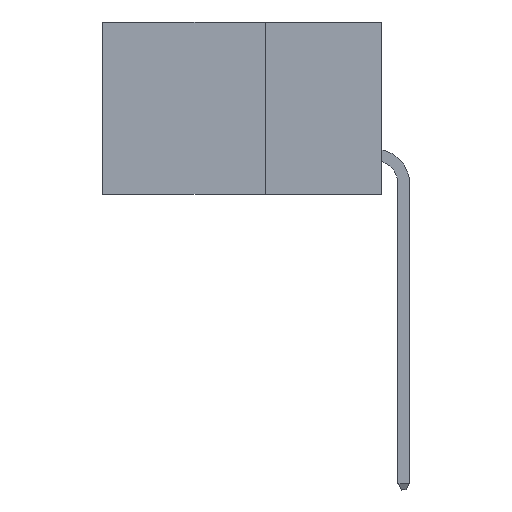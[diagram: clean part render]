
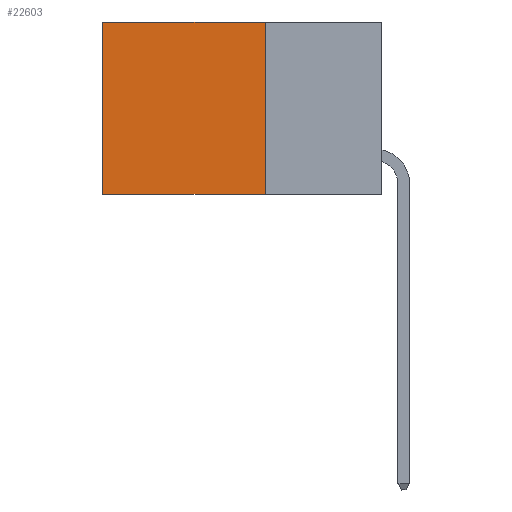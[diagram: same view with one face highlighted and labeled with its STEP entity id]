
A CAD part, left-side view. The second image highlights one B-rep face of the part: STEP entity #22603.
In plain terms, the highlighted planar face has unit normal (-1, 0, 0).
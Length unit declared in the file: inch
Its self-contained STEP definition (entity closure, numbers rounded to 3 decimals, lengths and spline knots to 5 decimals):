
#535 = VERTEX_POINT ( 'NONE', #19764 ) ;
#2864 = AXIS2_PLACEMENT_3D ( 'NONE', #6429, #10647, #20541 ) ;
#3341 = VECTOR ( 'NONE', #6551, 39.37008 ) ;
#3945 = VECTOR ( 'NONE', #6868, 39.37008 ) ;
#5042 = ORIENTED_EDGE ( 'NONE', *, *, #19455, .T. ) ;
#6429 = CARTESIAN_POINT ( 'NONE',  ( 0.2875, 0.25, 0. ) ) ;
#6497 = EDGE_CURVE ( 'NONE', #6923, #14140, #11892, .T. ) ;
#6551 = DIRECTION ( 'NONE',  ( 0., 0., -1. ) ) ;
#6698 = LINE ( 'NONE', #15968, #17803 ) ;
#6842 = CARTESIAN_POINT ( 'NONE',  ( 0.2875, 0.6, -0.37 ) ) ;
#6868 = DIRECTION ( 'NONE',  ( 0., 1., 0. ) ) ;
#6923 = VERTEX_POINT ( 'NONE', #15298 ) ;
#6982 = CARTESIAN_POINT ( 'NONE',  ( 0.2875, 0.25, 0. ) ) ;
#8754 = CARTESIAN_POINT ( 'NONE',  ( 0.2875, 0.25, 0. ) ) ;
#8800 = PLANE ( 'NONE',  #2864 ) ;
#9365 = CARTESIAN_POINT ( 'NONE',  ( 0.2875, 0.25, -0.37 ) ) ;
#10647 = DIRECTION ( 'NONE',  ( 1., 0., 0. ) ) ;
#11892 = LINE ( 'NONE', #9365, #3945 ) ;
#12185 = VERTEX_POINT ( 'NONE', #6982 ) ;
#14140 = VERTEX_POINT ( 'NONE', #6842 ) ;
#15125 = ORIENTED_EDGE ( 'NONE', *, *, #24851, .F. ) ;
#15298 = CARTESIAN_POINT ( 'NONE',  ( 0.2875, 0.25, -0.37 ) ) ;
#15968 = CARTESIAN_POINT ( 'NONE',  ( 0.2875, 0.25, 0. ) ) ;
#17476 = DIRECTION ( 'NONE',  ( 0., 0., -1. ) ) ;
#17803 = VECTOR ( 'NONE', #23981, 39.37008 ) ;
#19455 = EDGE_CURVE ( 'NONE', #535, #14140, #25986, .T. ) ;
#19461 = LINE ( 'NONE', #8754, #3341 ) ;
#19558 = FACE_OUTER_BOUND ( 'NONE', #22493, .T. ) ;
#19634 = EDGE_CURVE ( 'NONE', #12185, #535, #6698, .T. ) ;
#19764 = CARTESIAN_POINT ( 'NONE',  ( 0.2875, 0.6, 0. ) ) ;
#20541 = DIRECTION ( 'NONE',  ( 0., 0., -1. ) ) ;
#21256 = VECTOR ( 'NONE', #17476, 39.37008 ) ;
#21283 = ORIENTED_EDGE ( 'NONE', *, *, #19634, .T. ) ;
#21608 = CARTESIAN_POINT ( 'NONE',  ( 0.2875, 0.6, 0. ) ) ;
#22493 = EDGE_LOOP ( 'NONE', ( #5042, #26040, #15125, #21283 ) ) ;
#22603 = ADVANCED_FACE ( 'NONE', ( #19558 ), #8800, .F. ) ;
#23981 = DIRECTION ( 'NONE',  ( 0., 1., 0. ) ) ;
#24851 = EDGE_CURVE ( 'NONE', #12185, #6923, #19461, .T. ) ;
#25986 = LINE ( 'NONE', #21608, #21256 ) ;
#26040 = ORIENTED_EDGE ( 'NONE', *, *, #6497, .F. ) ;
